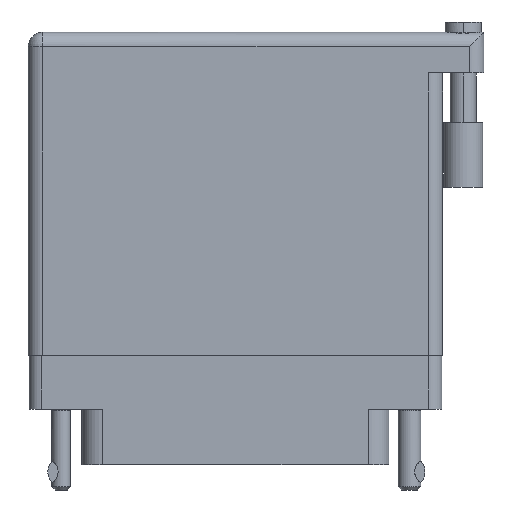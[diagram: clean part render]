
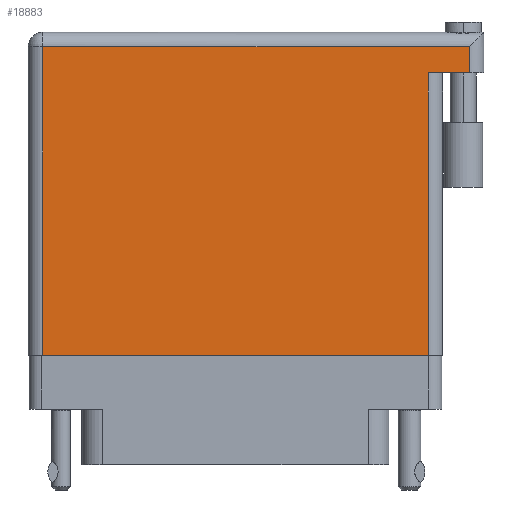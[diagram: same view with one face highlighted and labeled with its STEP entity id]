
A CAD part, front view. The second image highlights one B-rep face of the part: STEP entity #18883.
In plain terms, the highlighted face is planar.
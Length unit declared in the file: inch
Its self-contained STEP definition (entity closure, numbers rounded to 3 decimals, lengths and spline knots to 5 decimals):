
#295 = CARTESIAN_POINT ( 'NONE',  ( 1.938, 1.369, 0. ) ) ;
#3259 = VERTEX_POINT ( 'NONE', #36661 ) ;
#3302 = EDGE_CURVE ( 'NONE', #3259, #6105, #9205, .T. ) ;
#4778 = VERTEX_POINT ( 'NONE', #23299 ) ;
#5812 = DIRECTION ( 'NONE',  ( -1., 0., 0. ) ) ;
#6105 = VERTEX_POINT ( 'NONE', #30955 ) ;
#6513 = VECTOR ( 'NONE', #22482, 39.37008 ) ;
#6890 = LINE ( 'NONE', #295, #36361 ) ;
#7771 = PLANE ( 'NONE',  #47539 ) ;
#9205 = LINE ( 'NONE', #40205, #12690 ) ;
#10950 = DIRECTION ( 'NONE',  ( 0., 1., 0. ) ) ;
#12541 = LINE ( 'NONE', #16306, #47797 ) ;
#12549 = FACE_OUTER_BOUND ( 'NONE', #31046, .T. ) ;
#12690 = VECTOR ( 'NONE', #44054, 39.37008 ) ;
#13180 = VERTEX_POINT ( 'NONE', #24691 ) ;
#13403 = ORIENTED_EDGE ( 'NONE', *, *, #47722, .T. ) ;
#16306 = CARTESIAN_POINT ( 'NONE',  ( 2.138, 1.566, 0. ) ) ;
#18054 = VERTEX_POINT ( 'NONE', #47245 ) ;
#18883 = ADVANCED_FACE ( 'NONE', ( #12549 ), #7771, .F. ) ;
#19863 = ORIENTED_EDGE ( 'NONE', *, *, #22817, .T. ) ;
#21780 = VECTOR ( 'NONE', #39306, 39.37008 ) ;
#22364 = DIRECTION ( 'NONE',  ( 0., 0., -1. ) ) ;
#22482 = DIRECTION ( 'NONE',  ( 1., 0., 0. ) ) ;
#22534 = DIRECTION ( 'NONE',  ( -1., 0., 0. ) ) ;
#22817 = EDGE_CURVE ( 'NONE', #6105, #4778, #32575, .T. ) ;
#23299 = CARTESIAN_POINT ( 'NONE',  ( 1.938, 0., 0. ) ) ;
#23763 = ORIENTED_EDGE ( 'NONE', *, *, #41455, .F. ) ;
#24500 = CARTESIAN_POINT ( 'NONE',  ( 0., 1.496, 0. ) ) ;
#24691 = CARTESIAN_POINT ( 'NONE',  ( 2.138, 1.369, 0. ) ) ;
#25352 = ORIENTED_EDGE ( 'NONE', *, *, #26337, .T. ) ;
#26337 = EDGE_CURVE ( 'NONE', #13180, #18054, #12541, .T. ) ;
#27225 = ORIENTED_EDGE ( 'NONE', *, *, #3302, .T. ) ;
#27314 = EDGE_CURVE ( 'NONE', #18054, #3259, #35069, .T. ) ;
#29504 = CARTESIAN_POINT ( 'NONE',  ( 1.938, 1.369, 0. ) ) ;
#30955 = CARTESIAN_POINT ( 'NONE',  ( 0.07, 0., 0. ) ) ;
#31046 = EDGE_LOOP ( 'NONE', ( #19863, #13403, #23763, #25352, #43298, #27225 ) ) ;
#31151 = CARTESIAN_POINT ( 'NONE',  ( 2.208, 1.369, 0. ) ) ;
#32298 = VECTOR ( 'NONE', #5812, 39.37008 ) ;
#32575 = LINE ( 'NONE', #37465, #6513 ) ;
#35069 = LINE ( 'NONE', #24500, #21780 ) ;
#36361 = VECTOR ( 'NONE', #10950, 39.37008 ) ;
#36661 = CARTESIAN_POINT ( 'NONE',  ( 0.07, 1.496, 0. ) ) ;
#37465 = CARTESIAN_POINT ( 'NONE',  ( 0., 0., 0. ) ) ;
#37515 = CARTESIAN_POINT ( 'NONE',  ( 0., 1.566, 0. ) ) ;
#39306 = DIRECTION ( 'NONE',  ( -1., 0., 0. ) ) ;
#40205 = CARTESIAN_POINT ( 'NONE',  ( 0.07, 0., 0. ) ) ;
#41455 = EDGE_CURVE ( 'NONE', #13180, #42823, #47242, .T. ) ;
#42823 = VERTEX_POINT ( 'NONE', #29504 ) ;
#43298 = ORIENTED_EDGE ( 'NONE', *, *, #27314, .T. ) ;
#44054 = DIRECTION ( 'NONE',  ( 0., -1., 0. ) ) ;
#45951 = DIRECTION ( 'NONE',  ( 0., 1., 0. ) ) ;
#47242 = LINE ( 'NONE', #31151, #32298 ) ;
#47245 = CARTESIAN_POINT ( 'NONE',  ( 2.138, 1.496, 0. ) ) ;
#47539 = AXIS2_PLACEMENT_3D ( 'NONE', #37515, #22364, #22534 ) ;
#47722 = EDGE_CURVE ( 'NONE', #4778, #42823, #6890, .T. ) ;
#47797 = VECTOR ( 'NONE', #45951, 39.37008 ) ;
